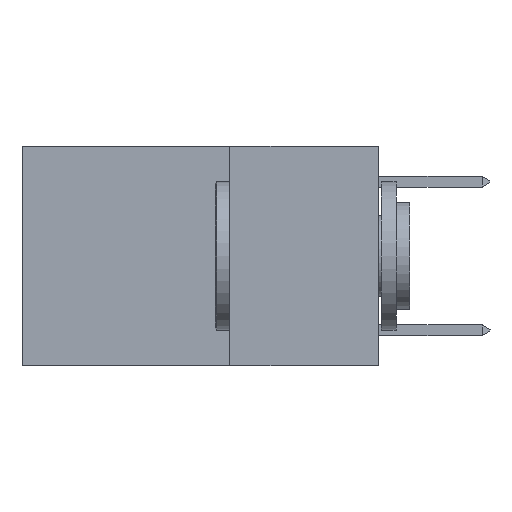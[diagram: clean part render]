
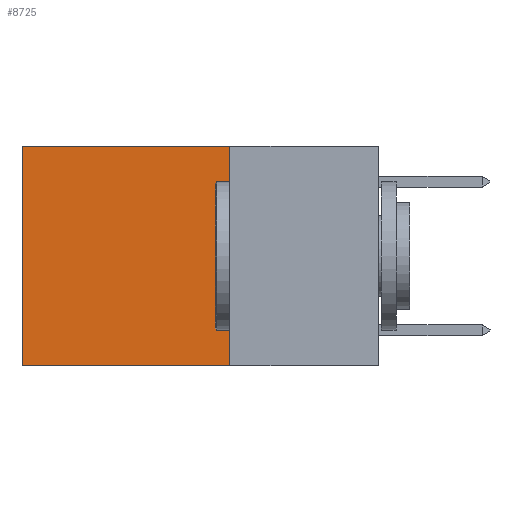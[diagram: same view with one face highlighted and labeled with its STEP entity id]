
A CAD part, left-side view. The second image highlights one B-rep face of the part: STEP entity #8725.
In plain terms, the highlighted planar face has unit normal (-1, 0, 0).
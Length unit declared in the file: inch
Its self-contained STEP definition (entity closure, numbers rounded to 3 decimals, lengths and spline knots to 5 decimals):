
#89 = VECTOR ( 'NONE', #11548, 39.37008 ) ;
#97 = VERTEX_POINT ( 'NONE', #2870 ) ;
#192 = PLANE ( 'NONE',  #7209 ) ;
#275 = DIRECTION ( 'NONE',  ( 1., 0., 0. ) ) ;
#386 = EDGE_CURVE ( 'NONE', #6527, #10010, #1032, .T. ) ;
#680 = EDGE_CURVE ( 'NONE', #97, #10483, #7122, .T. ) ;
#1032 = LINE ( 'NONE', #7052, #89 ) ;
#2681 = ORIENTED_EDGE ( 'NONE', *, *, #5551, .T. ) ;
#2870 = CARTESIAN_POINT ( 'NONE',  ( 0.2625, 0.6, 0. ) ) ;
#3440 = CARTESIAN_POINT ( 'NONE',  ( 0.2625, 0.25, -0.37 ) ) ;
#4113 = LINE ( 'NONE', #3440, #6362 ) ;
#4711 = ORIENTED_EDGE ( 'NONE', *, *, #386, .F. ) ;
#4744 = VECTOR ( 'NONE', #10257, 39.37008 ) ;
#5043 = EDGE_CURVE ( 'NONE', #10010, #10483, #4113, .T. ) ;
#5173 = ORIENTED_EDGE ( 'NONE', *, *, #5043, .F. ) ;
#5363 = CARTESIAN_POINT ( 'NONE',  ( 0.2625, 0.25, 0. ) ) ;
#5380 = FACE_OUTER_BOUND ( 'NONE', #11097, .T. ) ;
#5551 = EDGE_CURVE ( 'NONE', #6527, #97, #10188, .T. ) ;
#6150 = CARTESIAN_POINT ( 'NONE',  ( 0.2625, 0.25, 0. ) ) ;
#6362 = VECTOR ( 'NONE', #7043, 39.37008 ) ;
#6527 = VERTEX_POINT ( 'NONE', #5363 ) ;
#7043 = DIRECTION ( 'NONE',  ( 0., 1., 0. ) ) ;
#7052 = CARTESIAN_POINT ( 'NONE',  ( 0.2625, 0.25, 0. ) ) ;
#7122 = LINE ( 'NONE', #7451, #4744 ) ;
#7209 = AXIS2_PLACEMENT_3D ( 'NONE', #8295, #275, #9210 ) ;
#7451 = CARTESIAN_POINT ( 'NONE',  ( 0.2625, 0.6, 0. ) ) ;
#8295 = CARTESIAN_POINT ( 'NONE',  ( 0.2625, 0.25, 0. ) ) ;
#8350 = CARTESIAN_POINT ( 'NONE',  ( 0.2625, 0.6, -0.37 ) ) ;
#8725 = ADVANCED_FACE ( 'NONE', ( #5380 ), #192, .F. ) ;
#8936 = ORIENTED_EDGE ( 'NONE', *, *, #680, .T. ) ;
#9210 = DIRECTION ( 'NONE',  ( 0., 0., -1. ) ) ;
#10010 = VERTEX_POINT ( 'NONE', #10956 ) ;
#10188 = LINE ( 'NONE', #6150, #11032 ) ;
#10257 = DIRECTION ( 'NONE',  ( 0., 0., -1. ) ) ;
#10483 = VERTEX_POINT ( 'NONE', #8350 ) ;
#10740 = DIRECTION ( 'NONE',  ( 0., 1., 0. ) ) ;
#10956 = CARTESIAN_POINT ( 'NONE',  ( 0.2625, 0.25, -0.37 ) ) ;
#11032 = VECTOR ( 'NONE', #10740, 39.37008 ) ;
#11097 = EDGE_LOOP ( 'NONE', ( #8936, #5173, #4711, #2681 ) ) ;
#11548 = DIRECTION ( 'NONE',  ( 0., 0., -1. ) ) ;
